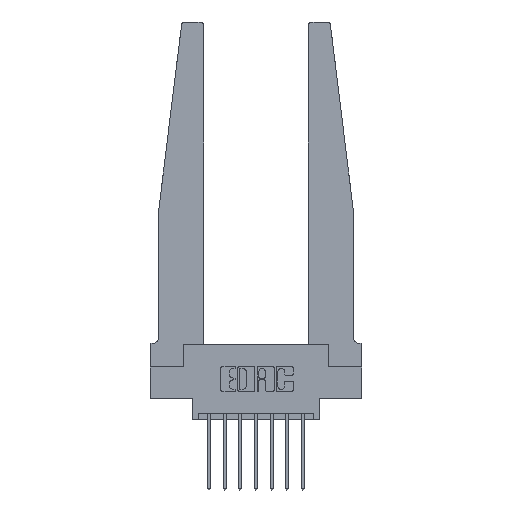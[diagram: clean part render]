
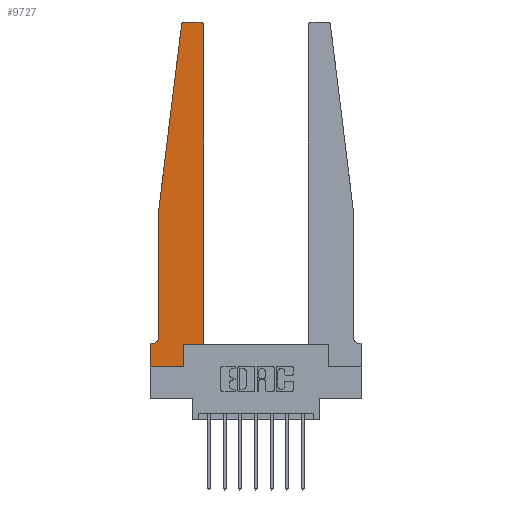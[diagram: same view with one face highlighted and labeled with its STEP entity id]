
A CAD part, top view. The second image highlights one B-rep face of the part: STEP entity #9727.
In plain terms, the highlighted planar face has unit normal (0, 0, 1).
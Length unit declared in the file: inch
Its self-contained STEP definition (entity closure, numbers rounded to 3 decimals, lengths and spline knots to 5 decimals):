
#255 = CIRCLE ( 'NONE', #2606, 0.03 ) ;
#339 = DIRECTION ( 'NONE',  ( -1., 0., 0. ) ) ;
#388 = CARTESIAN_POINT ( 'NONE',  ( 0., 0.1875, 0.37 ) ) ;
#391 = VERTEX_POINT ( 'NONE', #388 ) ;
#395 = VECTOR ( 'NONE', #11270, 39.37008 ) ;
#454 = VERTEX_POINT ( 'NONE', #1945 ) ;
#544 = EDGE_CURVE ( 'NONE', #3225, #8269, #255, .T. ) ;
#995 = EDGE_LOOP ( 'NONE', ( #6049, #3893, #3330, #4535, #12736, #9161, #1000, #9897, #13270, #12781, #7473, #6014 ) ) ;
#1000 = ORIENTED_EDGE ( 'NONE', *, *, #6633, .T. ) ;
#1225 = CIRCLE ( 'NONE', #9037, 0.03 ) ;
#1734 = VERTEX_POINT ( 'NONE', #9802 ) ;
#1785 = LINE ( 'NONE', #10596, #10078 ) ;
#1861 = CARTESIAN_POINT ( 'NONE',  ( 0.425, 0.18, 0.37 ) ) ;
#1945 = CARTESIAN_POINT ( 'NONE',  ( 0.2605, 0., 0.37 ) ) ;
#1974 = DIRECTION ( 'NONE',  ( -1., 0., 0. ) ) ;
#1994 = CARTESIAN_POINT ( 'NONE',  ( 0.27653, 2.75, 0.37 ) ) ;
#2004 = VECTOR ( 'NONE', #339, 39.37008 ) ;
#2606 = AXIS2_PLACEMENT_3D ( 'NONE', #10822, #2837, #10751 ) ;
#2626 = DIRECTION ( 'NONE',  ( 1., 0., 0. ) ) ;
#2752 = DIRECTION ( 'NONE',  ( -0.122, -0.992, 0. ) ) ;
#2773 = LINE ( 'NONE', #12772, #10244 ) ;
#2837 = DIRECTION ( 'NONE',  ( 0., 0., 1. ) ) ;
#3225 = VERTEX_POINT ( 'NONE', #14188 ) ;
#3330 = ORIENTED_EDGE ( 'NONE', *, *, #9316, .T. ) ;
#3355 = CARTESIAN_POINT ( 'NONE',  ( 0., 0., 0.37 ) ) ;
#3491 = VERTEX_POINT ( 'NONE', #13861 ) ;
#3518 = EDGE_CURVE ( 'NONE', #3491, #9194, #5499, .T. ) ;
#3893 = ORIENTED_EDGE ( 'NONE', *, *, #13654, .T. ) ;
#4067 = VERTEX_POINT ( 'NONE', #1994 ) ;
#4382 = EDGE_CURVE ( 'NONE', #9194, #391, #13346, .T. ) ;
#4535 = ORIENTED_EDGE ( 'NONE', *, *, #12152, .T. ) ;
#4637 = EDGE_CURVE ( 'NONE', #6453, #454, #2773, .T. ) ;
#4859 = VECTOR ( 'NONE', #9419, 39.37008 ) ;
#4924 = DIRECTION ( 'NONE',  ( 0., 0., -1. ) ) ;
#5093 = LINE ( 'NONE', #9370, #5124 ) ;
#5124 = VECTOR ( 'NONE', #6058, 39.37008 ) ;
#5499 = CIRCLE ( 'NONE', #7660, 0.05 ) ;
#5507 = CARTESIAN_POINT ( 'NONE',  ( 0.27653, 2.72, 0.37 ) ) ;
#5568 = VERTEX_POINT ( 'NONE', #8866 ) ;
#6014 = ORIENTED_EDGE ( 'NONE', *, *, #544, .T. ) ;
#6049 = ORIENTED_EDGE ( 'NONE', *, *, #10147, .T. ) ;
#6058 = DIRECTION ( 'NONE',  ( 1., 0., 0. ) ) ;
#6079 = PLANE ( 'NONE',  #13108 ) ;
#6294 = CARTESIAN_POINT ( 'NONE',  ( 0., 0.1875, 0.37 ) ) ;
#6373 = DIRECTION ( 'NONE',  ( 1., 0., 0. ) ) ;
#6453 = VERTEX_POINT ( 'NONE', #3355 ) ;
#6551 = DIRECTION ( 'NONE',  ( -1., 0., 0. ) ) ;
#6633 = EDGE_CURVE ( 'NONE', #391, #6453, #9132, .T. ) ;
#7162 = CARTESIAN_POINT ( 'NONE',  ( 0.25, 2.75, 0.37 ) ) ;
#7473 = ORIENTED_EDGE ( 'NONE', *, *, #14566, .T. ) ;
#7660 = AXIS2_PLACEMENT_3D ( 'NONE', #9437, #4924, #6551 ) ;
#7683 = VECTOR ( 'NONE', #1974, 39.37008 ) ;
#8269 = VERTEX_POINT ( 'NONE', #9563 ) ;
#8546 = CARTESIAN_POINT ( 'NONE',  ( 0.065, 1.25, 0.37 ) ) ;
#8682 = DIRECTION ( 'NONE',  ( 0., 1., 0. ) ) ;
#8866 = CARTESIAN_POINT ( 'NONE',  ( 0.2605, 0.18, 0.37 ) ) ;
#8978 = CARTESIAN_POINT ( 'NONE',  ( 0.2605, 0.18, 0.37 ) ) ;
#8998 = EDGE_CURVE ( 'NONE', #454, #5568, #12447, .T. ) ;
#9037 = AXIS2_PLACEMENT_3D ( 'NONE', #5507, #10157, #12167 ) ;
#9132 = LINE ( 'NONE', #10381, #11784 ) ;
#9161 = ORIENTED_EDGE ( 'NONE', *, *, #4382, .T. ) ;
#9194 = VERTEX_POINT ( 'NONE', #13614 ) ;
#9316 = EDGE_CURVE ( 'NONE', #9838, #1734, #1785, .T. ) ;
#9370 = CARTESIAN_POINT ( 'NONE',  ( 0.425, 0.18, 0.37 ) ) ;
#9419 = DIRECTION ( 'NONE',  ( 0., -1., 0. ) ) ;
#9437 = CARTESIAN_POINT ( 'NONE',  ( 0.015, 0.2375, 0.37 ) ) ;
#9563 = CARTESIAN_POINT ( 'NONE',  ( 0.395, 2.75, 0.37 ) ) ;
#9727 = ADVANCED_FACE ( 'NONE', ( #10655 ), #6079, .T. ) ;
#9802 = CARTESIAN_POINT ( 'NONE',  ( 0.065, 1.25, 0.37 ) ) ;
#9838 = VERTEX_POINT ( 'NONE', #11096 ) ;
#9897 = ORIENTED_EDGE ( 'NONE', *, *, #4637, .T. ) ;
#10078 = VECTOR ( 'NONE', #2752, 39.37008 ) ;
#10112 = VECTOR ( 'NONE', #8682, 39.37008 ) ;
#10122 = EDGE_CURVE ( 'NONE', #5568, #14299, #5093, .T. ) ;
#10147 = EDGE_CURVE ( 'NONE', #8269, #4067, #13874, .T. ) ;
#10157 = DIRECTION ( 'NONE',  ( 0., 0., 1. ) ) ;
#10244 = VECTOR ( 'NONE', #2626, 39.37008 ) ;
#10381 = CARTESIAN_POINT ( 'NONE',  ( 0., 0., 0.37 ) ) ;
#10455 = DIRECTION ( 'NONE',  ( 0., -1., 0. ) ) ;
#10596 = CARTESIAN_POINT ( 'NONE',  ( 0.065, 1.25, 0.37 ) ) ;
#10655 = FACE_OUTER_BOUND ( 'NONE', #995, .T. ) ;
#10751 = DIRECTION ( 'NONE',  ( 1., 0., 0. ) ) ;
#10822 = CARTESIAN_POINT ( 'NONE',  ( 0.395, 2.72, 0.37 ) ) ;
#11096 = CARTESIAN_POINT ( 'NONE',  ( 0.24675, 2.72367, 0.37 ) ) ;
#11270 = DIRECTION ( 'NONE',  ( 0., 1., 0. ) ) ;
#11784 = VECTOR ( 'NONE', #10455, 39.37008 ) ;
#12152 = EDGE_CURVE ( 'NONE', #1734, #3491, #13993, .T. ) ;
#12167 = DIRECTION ( 'NONE',  ( 1., 0., 0. ) ) ;
#12254 = CARTESIAN_POINT ( 'NONE',  ( 0.065, 0.1875, 0.37 ) ) ;
#12447 = LINE ( 'NONE', #8978, #395 ) ;
#12736 = ORIENTED_EDGE ( 'NONE', *, *, #3518, .T. ) ;
#12772 = CARTESIAN_POINT ( 'NONE',  ( 0., 0., 0.37 ) ) ;
#12781 = ORIENTED_EDGE ( 'NONE', *, *, #10122, .T. ) ;
#13108 = AXIS2_PLACEMENT_3D ( 'NONE', #6294, #13901, #6373 ) ;
#13270 = ORIENTED_EDGE ( 'NONE', *, *, #8998, .T. ) ;
#13346 = LINE ( 'NONE', #12254, #7683 ) ;
#13614 = CARTESIAN_POINT ( 'NONE',  ( 0.015, 0.1875, 0.37 ) ) ;
#13654 = EDGE_CURVE ( 'NONE', #4067, #9838, #1225, .T. ) ;
#13771 = CARTESIAN_POINT ( 'NONE',  ( 0.425, 0.18, 0.37 ) ) ;
#13861 = CARTESIAN_POINT ( 'NONE',  ( 0.065, 0.2375, 0.37 ) ) ;
#13874 = LINE ( 'NONE', #7162, #2004 ) ;
#13901 = DIRECTION ( 'NONE',  ( 0., 0., 1. ) ) ;
#13993 = LINE ( 'NONE', #8546, #4859 ) ;
#14188 = CARTESIAN_POINT ( 'NONE',  ( 0.425, 2.72, 0.37 ) ) ;
#14299 = VERTEX_POINT ( 'NONE', #13771 ) ;
#14301 = LINE ( 'NONE', #1861, #10112 ) ;
#14566 = EDGE_CURVE ( 'NONE', #14299, #3225, #14301, .T. ) ;
